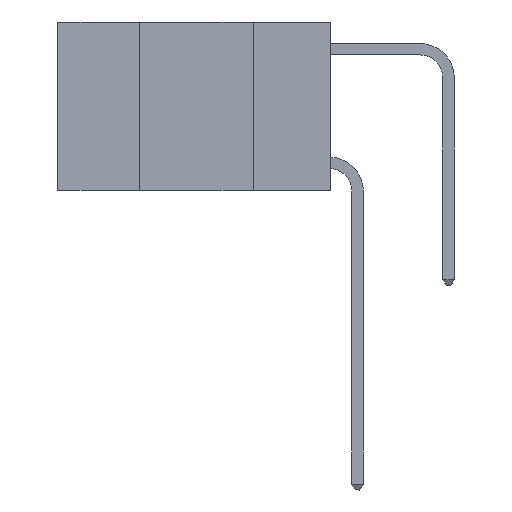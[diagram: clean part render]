
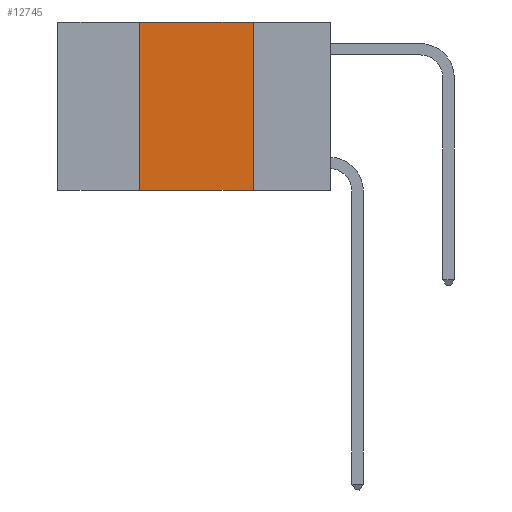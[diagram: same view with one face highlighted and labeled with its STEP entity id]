
A CAD part, left-side view. The second image highlights one B-rep face of the part: STEP entity #12745.
In plain terms, the highlighted planar face has unit normal (-1, 0, 0).
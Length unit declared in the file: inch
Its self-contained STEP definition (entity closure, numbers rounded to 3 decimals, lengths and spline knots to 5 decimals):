
#1275 = CARTESIAN_POINT ( 'NONE',  ( 0., 0.6, 0. ) ) ;
#2378 = DIRECTION ( 'NONE',  ( 0., 0., 1. ) ) ;
#3778 = EDGE_CURVE ( 'NONE', #5459, #26672, #4951, .T. ) ;
#3829 = DIRECTION ( 'NONE',  ( 1., 0., 0. ) ) ;
#4813 = CARTESIAN_POINT ( 'NONE',  ( 0., 0.17, -0.37 ) ) ;
#4951 = LINE ( 'NONE', #15485, #24541 ) ;
#5459 = VERTEX_POINT ( 'NONE', #28183 ) ;
#6483 = LINE ( 'NONE', #25263, #33291 ) ;
#6674 = VERTEX_POINT ( 'NONE', #18427 ) ;
#7300 = CARTESIAN_POINT ( 'NONE',  ( 0., 0.42, 0. ) ) ;
#10836 = CARTESIAN_POINT ( 'NONE',  ( 0., 0.6, -0.37 ) ) ;
#11890 = VECTOR ( 'NONE', #14942, 39.37008 ) ;
#12745 = ADVANCED_FACE ( 'NONE', ( #14036 ), #19339, .F. ) ;
#12854 = LINE ( 'NONE', #32982, #11890 ) ;
#14036 = FACE_OUTER_BOUND ( 'NONE', #15146, .T. ) ;
#14942 = DIRECTION ( 'NONE',  ( 0., 0., -1. ) ) ;
#15146 = EDGE_LOOP ( 'NONE', ( #16559, #21260, #19849, #16059 ) ) ;
#15485 = CARTESIAN_POINT ( 'NONE',  ( 0., 0.42, 0. ) ) ;
#16059 = ORIENTED_EDGE ( 'NONE', *, *, #24676, .T. ) ;
#16559 = ORIENTED_EDGE ( 'NONE', *, *, #17834, .F. ) ;
#16677 = DIRECTION ( 'NONE',  ( 0., -1., 0. ) ) ;
#17834 = EDGE_CURVE ( 'NONE', #6674, #20953, #12854, .T. ) ;
#18427 = CARTESIAN_POINT ( 'NONE',  ( 0., 0.17, 0. ) ) ;
#18915 = LINE ( 'NONE', #10836, #20402 ) ;
#19339 = PLANE ( 'NONE',  #29797 ) ;
#19849 = ORIENTED_EDGE ( 'NONE', *, *, #3778, .F. ) ;
#20402 = VECTOR ( 'NONE', #16677, 39.37008 ) ;
#20953 = VERTEX_POINT ( 'NONE', #4813 ) ;
#21260 = ORIENTED_EDGE ( 'NONE', *, *, #31974, .F. ) ;
#24541 = VECTOR ( 'NONE', #2378, 39.37008 ) ;
#24676 = EDGE_CURVE ( 'NONE', #5459, #20953, #18915, .T. ) ;
#25263 = CARTESIAN_POINT ( 'NONE',  ( 0., 0.6, 0. ) ) ;
#26672 = VERTEX_POINT ( 'NONE', #7300 ) ;
#28183 = CARTESIAN_POINT ( 'NONE',  ( 0., 0.42, -0.37 ) ) ;
#29797 = AXIS2_PLACEMENT_3D ( 'NONE', #1275, #3829, #29827 ) ;
#29827 = DIRECTION ( 'NONE',  ( 0., 0., -1. ) ) ;
#30411 = DIRECTION ( 'NONE',  ( 0., -1., 0. ) ) ;
#31974 = EDGE_CURVE ( 'NONE', #26672, #6674, #6483, .T. ) ;
#32982 = CARTESIAN_POINT ( 'NONE',  ( 0., 0.17, 0. ) ) ;
#33291 = VECTOR ( 'NONE', #30411, 39.37008 ) ;
